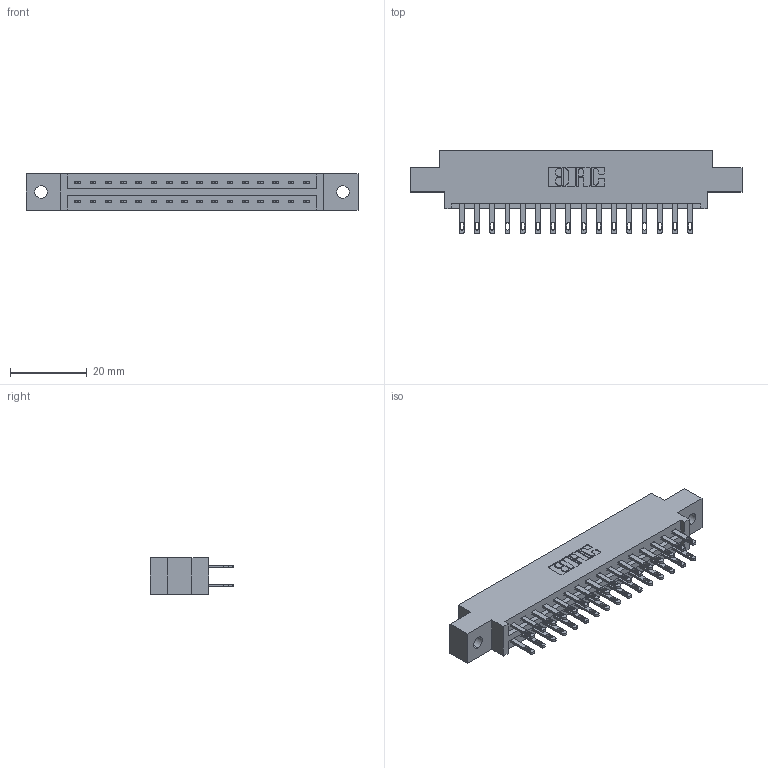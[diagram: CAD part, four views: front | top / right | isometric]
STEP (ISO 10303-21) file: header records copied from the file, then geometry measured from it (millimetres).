
FILE_DESCRIPTION (( 'STEP AP203' ), '1' );
FILE_NAME ('887-032-500-802.STEP', '2020-09-20T21:16:06', ( '' ), ( '' ), 'SwSTEP 2.0', 'SolidWorks 2020', '' );
FILE_SCHEMA (( 'CONFIG_CONTROL_DESIGN' ));
Length unit declared in the file: inch
Products named in the file (3): 837 Part_0.170 Offset - 0.128 Dia; 887-032-500-802; 345-292-001_345-293-100
Assembly tree (33 placements, depth 2):
  887-032-500-802
    837 Part_0.170 Offset - 0.128 Dia
    345-292-001_345-293-100  x32
Bounding box: 86.41 x 21.85 x 9.4 mm (x, y, z)
Volume: 8704.2 mm3; surface area: 9777.7 mm2
Topology: 33 solids, 33 shells, 1718 faces, 5219 edges, 3478 vertices
Faces by surface type: plane 1098, cylinder 620
Entity records: 15833 total; most frequent: CARTESIAN_POINT 2690, ORIENTED_EDGE 2626, DIRECTION 2337, EDGE_CURVE 1313, LINE 1181, VECTOR 1181, VERTEX_POINT 874, AXIS2_PLACEMENT_3D 578
